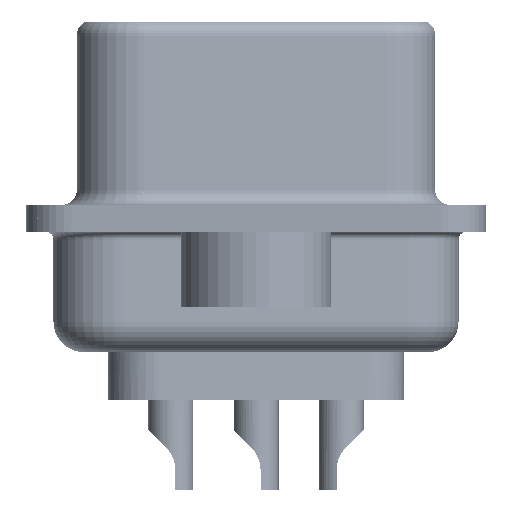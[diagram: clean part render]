
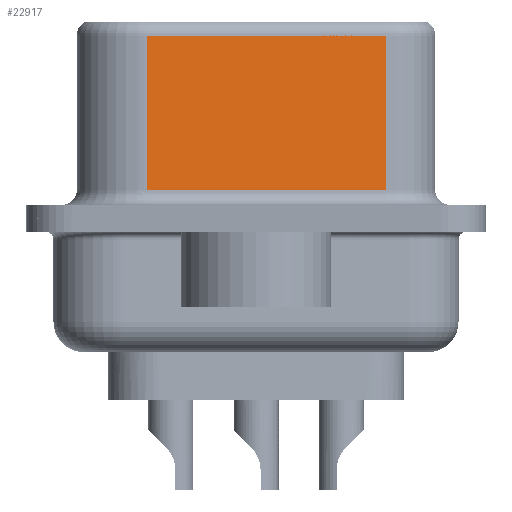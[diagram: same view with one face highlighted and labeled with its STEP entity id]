
A CAD part, left-side view. The second image highlights one B-rep face of the part: STEP entity #22917.
In plain terms, the highlighted planar face has unit normal (-0.985, -0.174, 0).
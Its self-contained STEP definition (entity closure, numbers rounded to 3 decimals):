
#411 = LINE ( 'NONE', #27704, #24994 ) ;
#576 = DIRECTION ( 'NONE',  ( 0.174, -0.985, 0. ) ) ;
#1268 = DIRECTION ( 'NONE',  ( -0.174, 0.985, 0. ) ) ;
#1775 = CARTESIAN_POINT ( 'NONE',  ( 3.73, 3.628, 6.55 ) ) ;
#2427 = ORIENTED_EDGE ( 'NONE', *, *, #6600, .T. ) ;
#2895 = VERTEX_POINT ( 'NONE', #29521 ) ;
#3835 = ORIENTED_EDGE ( 'NONE', *, *, #13918, .F. ) ;
#4318 = DIRECTION ( 'NONE',  ( 0., 0., -1. ) ) ;
#5171 = VECTOR ( 'NONE', #13630, 1000. ) ;
#6184 = FACE_OUTER_BOUND ( 'NONE', #25840, .T. ) ;
#6600 = EDGE_CURVE ( 'NONE', #12733, #9346, #28748, .T. ) ;
#6786 = CARTESIAN_POINT ( 'NONE',  ( 5.132, -4.322, 6.55 ) ) ;
#7930 = EDGE_CURVE ( 'NONE', #9346, #25097, #411, .T. ) ;
#9220 = CARTESIAN_POINT ( 'NONE',  ( 3.73, 3.628, 0.95 ) ) ;
#9346 = VERTEX_POINT ( 'NONE', #9220 ) ;
#10213 = VECTOR ( 'NONE', #4318, 1000. ) ;
#11838 = VECTOR ( 'NONE', #19247, 1000. ) ;
#12733 = VERTEX_POINT ( 'NONE', #25728 ) ;
#13630 = DIRECTION ( 'NONE',  ( -0.174, 0.985, 0. ) ) ;
#13918 = EDGE_CURVE ( 'NONE', #2895, #25097, #24428, .T. ) ;
#15266 = EDGE_CURVE ( 'NONE', #2895, #12733, #20840, .T. ) ;
#16592 = DIRECTION ( 'NONE',  ( 0.985, 0.174, 0. ) ) ;
#19247 = DIRECTION ( 'NONE',  ( 0., 0., -1. ) ) ;
#20840 = LINE ( 'NONE', #30986, #5171 ) ;
#22556 = ORIENTED_EDGE ( 'NONE', *, *, #7930, .T. ) ;
#22917 = ADVANCED_FACE ( 'NONE', ( #6184 ), #26269, .F. ) ;
#24428 = LINE ( 'NONE', #6786, #10213 ) ;
#24994 = VECTOR ( 'NONE', #576, 1000. ) ;
#25097 = VERTEX_POINT ( 'NONE', #29781 ) ;
#25728 = CARTESIAN_POINT ( 'NONE',  ( 3.73, 3.628, 6.1 ) ) ;
#25840 = EDGE_LOOP ( 'NONE', ( #3835, #28013, #2427, #22556 ) ) ;
#26269 = PLANE ( 'NONE',  #28046 ) ;
#27704 = CARTESIAN_POINT ( 'NONE',  ( 5.132, -4.322, 0.95 ) ) ;
#28013 = ORIENTED_EDGE ( 'NONE', *, *, #15266, .T. ) ;
#28046 = AXIS2_PLACEMENT_3D ( 'NONE', #31485, #16592, #1268 ) ;
#28748 = LINE ( 'NONE', #1775, #11838 ) ;
#29521 = CARTESIAN_POINT ( 'NONE',  ( 5.132, -4.322, 6.1 ) ) ;
#29781 = CARTESIAN_POINT ( 'NONE',  ( 5.132, -4.322, 0.95 ) ) ;
#30986 = CARTESIAN_POINT ( 'NONE',  ( 5.132, -4.322, 6.1 ) ) ;
#31485 = CARTESIAN_POINT ( 'NONE',  ( 5.132, -4.322, 6.55 ) ) ;
